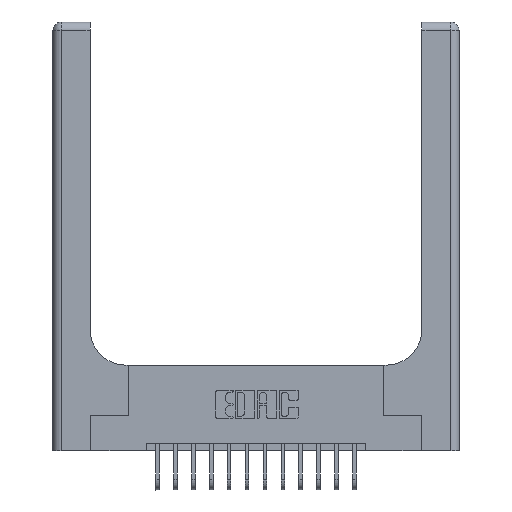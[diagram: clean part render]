
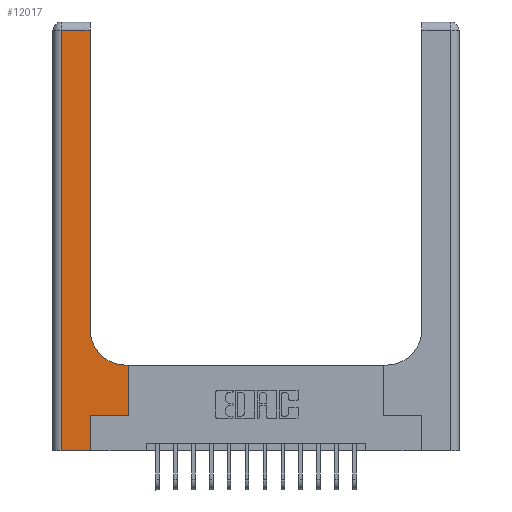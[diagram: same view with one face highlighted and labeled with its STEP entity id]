
A CAD part, top view. The second image highlights one B-rep face of the part: STEP entity #12017.
In plain terms, the highlighted planar face has unit normal (0, 0, 1).
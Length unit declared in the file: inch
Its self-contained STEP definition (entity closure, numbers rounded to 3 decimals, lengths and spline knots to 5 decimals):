
#120 = AXIS2_PLACEMENT_3D ( 'NONE', #7478, #14723, #17616 ) ;
#449 = VECTOR ( 'NONE', #18192, 39.37008 ) ;
#720 = VERTEX_POINT ( 'NONE', #18383 ) ;
#751 = EDGE_CURVE ( 'NONE', #720, #919, #1850, .T. ) ;
#762 = CARTESIAN_POINT ( 'NONE',  ( 0.06, 3., 0.37 ) ) ;
#919 = VERTEX_POINT ( 'NONE', #7916 ) ;
#1152 = EDGE_CURVE ( 'NONE', #6744, #6230, #17570, .T. ) ;
#1195 = CARTESIAN_POINT ( 'NONE',  ( 0.26, 0.85, 0.37 ) ) ;
#1232 = EDGE_LOOP ( 'NONE', ( #18673, #15010, #4744, #6888, #17420, #18799, #18135, #12966, #8537 ) ) ;
#1489 = CARTESIAN_POINT ( 'NONE',  ( 0.26, 2.94, 0.37 ) ) ;
#1822 = CARTESIAN_POINT ( 'NONE',  ( 0.51, 0.6, 0.37 ) ) ;
#1850 = LINE ( 'NONE', #14022, #5056 ) ;
#1854 = CARTESIAN_POINT ( 'NONE',  ( 0.26, 3., 0.37 ) ) ;
#1963 = VERTEX_POINT ( 'NONE', #1489 ) ;
#2185 = CARTESIAN_POINT ( 'NONE',  ( 0., 2.94, 0.37 ) ) ;
#2191 = CARTESIAN_POINT ( 'NONE',  ( 0., 0., 0.37 ) ) ;
#2299 = EDGE_CURVE ( 'NONE', #17253, #1963, #8462, .T. ) ;
#2693 = LINE ( 'NONE', #762, #449 ) ;
#3381 = LINE ( 'NONE', #8850, #3831 ) ;
#3748 = EDGE_CURVE ( 'NONE', #10135, #17253, #18382, .T. ) ;
#3831 = VECTOR ( 'NONE', #17646, 39.37008 ) ;
#3876 = LINE ( 'NONE', #8058, #16140 ) ;
#4257 = VERTEX_POINT ( 'NONE', #14852 ) ;
#4744 = ORIENTED_EDGE ( 'NONE', *, *, #8039, .T. ) ;
#5056 = VECTOR ( 'NONE', #15815, 39.37008 ) ;
#6173 = DIRECTION ( 'NONE',  ( -1., 0., 0. ) ) ;
#6230 = VERTEX_POINT ( 'NONE', #13390 ) ;
#6275 = DIRECTION ( 'NONE',  ( 0., 1., 0. ) ) ;
#6379 = CARTESIAN_POINT ( 'NONE',  ( 0.06, 2.94, 0.37 ) ) ;
#6496 = DIRECTION ( 'NONE',  ( -1., 0., 0. ) ) ;
#6521 = DIRECTION ( 'NONE',  ( 0., 1., 0. ) ) ;
#6744 = VERTEX_POINT ( 'NONE', #11045 ) ;
#6888 = ORIENTED_EDGE ( 'NONE', *, *, #1152, .T. ) ;
#7478 = CARTESIAN_POINT ( 'NONE',  ( 0.51, 0.85, 0.37 ) ) ;
#7606 = VECTOR ( 'NONE', #6496, 39.37008 ) ;
#7916 = CARTESIAN_POINT ( 'NONE',  ( 0.528, 0.25, 0.37 ) ) ;
#8039 = EDGE_CURVE ( 'NONE', #13426, #6744, #2693, .T. ) ;
#8058 = CARTESIAN_POINT ( 'NONE',  ( 0.528, 0.25, 0.37 ) ) ;
#8462 = LINE ( 'NONE', #1854, #18193 ) ;
#8537 = ORIENTED_EDGE ( 'NONE', *, *, #3748, .T. ) ;
#8850 = CARTESIAN_POINT ( 'NONE',  ( 0.265, 0., 0.37 ) ) ;
#8883 = EDGE_CURVE ( 'NONE', #6230, #720, #3381, .T. ) ;
#9584 = CARTESIAN_POINT ( 'NONE',  ( 0.26, 0.6, 0.37 ) ) ;
#10135 = VERTEX_POINT ( 'NONE', #1822 ) ;
#11045 = CARTESIAN_POINT ( 'NONE',  ( 0.06, 0., 0.37 ) ) ;
#11811 = FACE_OUTER_BOUND ( 'NONE', #1232, .T. ) ;
#11977 = DIRECTION ( 'NONE',  ( 0., 0., -1. ) ) ;
#12017 = ADVANCED_FACE ( 'NONE', ( #11811 ), #13208, .F. ) ;
#12573 = AXIS2_PLACEMENT_3D ( 'NONE', #17619, #11977, #6173 ) ;
#12966 = ORIENTED_EDGE ( 'NONE', *, *, #15674, .T. ) ;
#13208 = PLANE ( 'NONE',  #12573 ) ;
#13390 = CARTESIAN_POINT ( 'NONE',  ( 0.265, 0., 0.37 ) ) ;
#13426 = VERTEX_POINT ( 'NONE', #6379 ) ;
#13751 = DIRECTION ( 'NONE',  ( -1., 0., 0. ) ) ;
#13936 = DIRECTION ( 'NONE',  ( 1., 0., 0. ) ) ;
#14022 = CARTESIAN_POINT ( 'NONE',  ( 0.265, 0.25, 0.37 ) ) ;
#14723 = DIRECTION ( 'NONE',  ( 0., 0., -1. ) ) ;
#14812 = VECTOR ( 'NONE', #13936, 39.37008 ) ;
#14842 = LINE ( 'NONE', #9584, #16218 ) ;
#14852 = CARTESIAN_POINT ( 'NONE',  ( 0.528, 0.6, 0.37 ) ) ;
#15010 = ORIENTED_EDGE ( 'NONE', *, *, #16371, .T. ) ;
#15674 = EDGE_CURVE ( 'NONE', #4257, #10135, #14842, .T. ) ;
#15815 = DIRECTION ( 'NONE',  ( 1., 0., 0. ) ) ;
#16140 = VECTOR ( 'NONE', #6521, 39.37008 ) ;
#16218 = VECTOR ( 'NONE', #13751, 39.37008 ) ;
#16371 = EDGE_CURVE ( 'NONE', #1963, #13426, #16433, .T. ) ;
#16433 = LINE ( 'NONE', #2185, #7606 ) ;
#17253 = VERTEX_POINT ( 'NONE', #1195 ) ;
#17420 = ORIENTED_EDGE ( 'NONE', *, *, #8883, .T. ) ;
#17570 = LINE ( 'NONE', #2191, #14812 ) ;
#17616 = DIRECTION ( 'NONE',  ( 1., 0., 0. ) ) ;
#17619 = CARTESIAN_POINT ( 'NONE',  ( 0., 3., 0.37 ) ) ;
#17646 = DIRECTION ( 'NONE',  ( 0., 1., 0. ) ) ;
#17654 = EDGE_CURVE ( 'NONE', #919, #4257, #3876, .T. ) ;
#18135 = ORIENTED_EDGE ( 'NONE', *, *, #17654, .T. ) ;
#18192 = DIRECTION ( 'NONE',  ( 0., -1., 0. ) ) ;
#18193 = VECTOR ( 'NONE', #6275, 39.37008 ) ;
#18382 = CIRCLE ( 'NONE', #120, 0.25 ) ;
#18383 = CARTESIAN_POINT ( 'NONE',  ( 0.265, 0.25, 0.37 ) ) ;
#18673 = ORIENTED_EDGE ( 'NONE', *, *, #2299, .T. ) ;
#18799 = ORIENTED_EDGE ( 'NONE', *, *, #751, .T. ) ;
